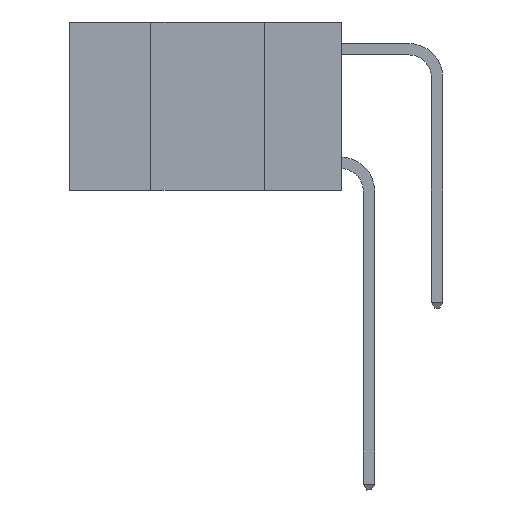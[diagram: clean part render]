
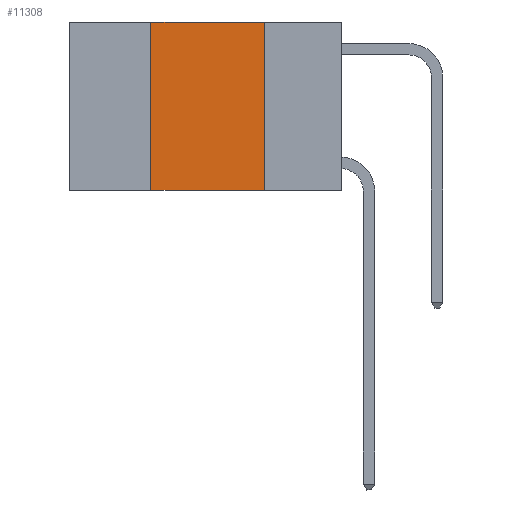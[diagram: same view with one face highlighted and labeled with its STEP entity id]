
A CAD part, left-side view. The second image highlights one B-rep face of the part: STEP entity #11308.
In plain terms, the highlighted planar face has unit normal (-1, 0, 0).
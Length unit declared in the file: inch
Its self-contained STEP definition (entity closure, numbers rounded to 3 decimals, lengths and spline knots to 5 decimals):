
#218 = ORIENTED_EDGE ( 'NONE', *, *, #10860, .T. ) ;
#622 = DIRECTION ( 'NONE',  ( 0., -1., 0. ) ) ;
#865 = VECTOR ( 'NONE', #4514, 39.37008 ) ;
#1413 = VERTEX_POINT ( 'NONE', #8049 ) ;
#2184 = CARTESIAN_POINT ( 'NONE',  ( 0., 0.6, 0. ) ) ;
#2577 = EDGE_CURVE ( 'NONE', #5790, #1413, #9525, .T. ) ;
#3263 = ORIENTED_EDGE ( 'NONE', *, *, #10125, .F. ) ;
#3327 = FACE_OUTER_BOUND ( 'NONE', #8867, .T. ) ;
#3399 = ORIENTED_EDGE ( 'NONE', *, *, #2577, .F. ) ;
#3551 = CARTESIAN_POINT ( 'NONE',  ( 0., 0.6, 0. ) ) ;
#3791 = CARTESIAN_POINT ( 'NONE',  ( 0., 0.42, -0.37 ) ) ;
#3883 = ORIENTED_EDGE ( 'NONE', *, *, #9017, .F. ) ;
#4180 = PLANE ( 'NONE',  #5269 ) ;
#4514 = DIRECTION ( 'NONE',  ( 0., -1., 0. ) ) ;
#5041 = CARTESIAN_POINT ( 'NONE',  ( 0., 0.42, 0. ) ) ;
#5131 = DIRECTION ( 'NONE',  ( 0., 0., -1. ) ) ;
#5159 = CARTESIAN_POINT ( 'NONE',  ( 0., 0.17, 0. ) ) ;
#5269 = AXIS2_PLACEMENT_3D ( 'NONE', #2184, #10637, #5131 ) ;
#5295 = VECTOR ( 'NONE', #622, 39.37008 ) ;
#5589 = LINE ( 'NONE', #11935, #5295 ) ;
#5790 = VERTEX_POINT ( 'NONE', #3791 ) ;
#5994 = DIRECTION ( 'NONE',  ( 0., 0., 1. ) ) ;
#6030 = LINE ( 'NONE', #3551, #865 ) ;
#6929 = CARTESIAN_POINT ( 'NONE',  ( 0., 0.17, 0. ) ) ;
#7057 = VECTOR ( 'NONE', #5994, 39.37008 ) ;
#7236 = VERTEX_POINT ( 'NONE', #11444 ) ;
#8049 = CARTESIAN_POINT ( 'NONE',  ( 0., 0.42, 0. ) ) ;
#8291 = VECTOR ( 'NONE', #9728, 39.37008 ) ;
#8593 = LINE ( 'NONE', #5159, #8291 ) ;
#8790 = VERTEX_POINT ( 'NONE', #6929 ) ;
#8867 = EDGE_LOOP ( 'NONE', ( #3263, #3883, #3399, #218 ) ) ;
#9017 = EDGE_CURVE ( 'NONE', #1413, #8790, #6030, .T. ) ;
#9525 = LINE ( 'NONE', #5041, #7057 ) ;
#9728 = DIRECTION ( 'NONE',  ( 0., 0., -1. ) ) ;
#10125 = EDGE_CURVE ( 'NONE', #8790, #7236, #8593, .T. ) ;
#10637 = DIRECTION ( 'NONE',  ( 1., 0., 0. ) ) ;
#10860 = EDGE_CURVE ( 'NONE', #5790, #7236, #5589, .T. ) ;
#11308 = ADVANCED_FACE ( 'NONE', ( #3327 ), #4180, .F. ) ;
#11444 = CARTESIAN_POINT ( 'NONE',  ( 0., 0.17, -0.37 ) ) ;
#11935 = CARTESIAN_POINT ( 'NONE',  ( 0., 0.6, -0.37 ) ) ;
